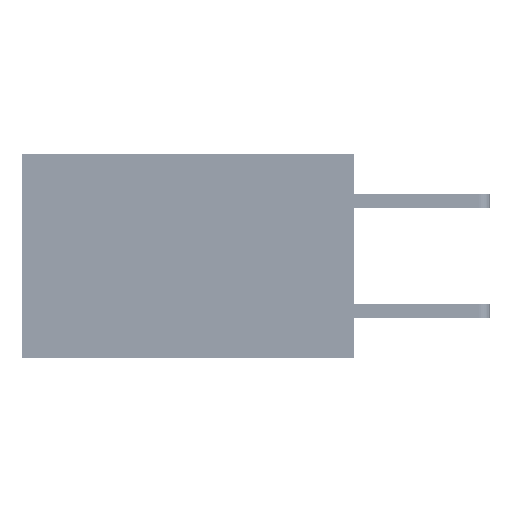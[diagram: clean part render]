
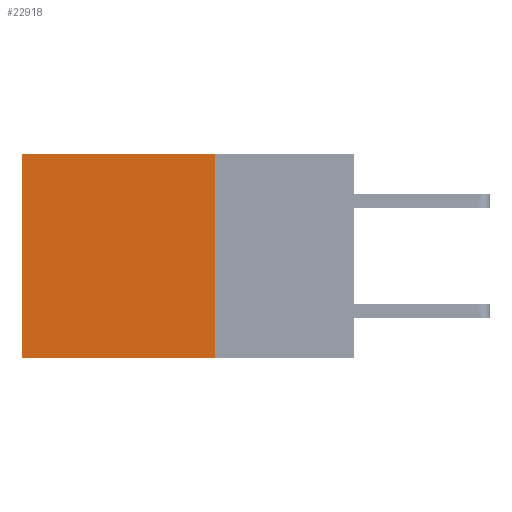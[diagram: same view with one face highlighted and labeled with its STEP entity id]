
A CAD part, left-side view. The second image highlights one B-rep face of the part: STEP entity #22918.
In plain terms, the highlighted planar face has unit normal (-1, 0, 0).
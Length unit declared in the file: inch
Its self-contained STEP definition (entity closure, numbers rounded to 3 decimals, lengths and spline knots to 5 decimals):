
#1767 = VECTOR ( 'NONE', #21073, 39.37008 ) ;
#2287 = VERTEX_POINT ( 'NONE', #46530 ) ;
#2504 = CARTESIAN_POINT ( 'NONE',  ( 0.2875, 0.6, 0. ) ) ;
#5168 = PLANE ( 'NONE',  #28228 ) ;
#5195 = LINE ( 'NONE', #44268, #1767 ) ;
#5915 = DIRECTION ( 'NONE',  ( 1., 0., 0. ) ) ;
#6363 = ORIENTED_EDGE ( 'NONE', *, *, #23171, .T. ) ;
#7543 = ORIENTED_EDGE ( 'NONE', *, *, #28439, .T. ) ;
#7754 = CARTESIAN_POINT ( 'NONE',  ( 0.2875, 0.25, 0. ) ) ;
#10419 = VERTEX_POINT ( 'NONE', #2504 ) ;
#11437 = DIRECTION ( 'NONE',  ( 0., 1., 0. ) ) ;
#13865 = DIRECTION ( 'NONE',  ( 0., 1., 0. ) ) ;
#14761 = VECTOR ( 'NONE', #13865, 39.37008 ) ;
#18818 = CARTESIAN_POINT ( 'NONE',  ( 0.2875, 0.25, 0. ) ) ;
#19521 = CARTESIAN_POINT ( 'NONE',  ( 0.2875, 0.6, -0.37 ) ) ;
#20540 = CARTESIAN_POINT ( 'NONE',  ( 0.2875, 0.25, 0. ) ) ;
#21041 = FACE_OUTER_BOUND ( 'NONE', #22159, .T. ) ;
#21073 = DIRECTION ( 'NONE',  ( 0., 0., -1. ) ) ;
#22159 = EDGE_LOOP ( 'NONE', ( #7543, #45518, #33792, #6363 ) ) ;
#22600 = EDGE_CURVE ( 'NONE', #38400, #2287, #37507, .T. ) ;
#22918 = ADVANCED_FACE ( 'NONE', ( #21041 ), #5168, .F. ) ;
#23171 = EDGE_CURVE ( 'NONE', #38400, #10419, #34877, .T. ) ;
#23288 = CARTESIAN_POINT ( 'NONE',  ( 0.2875, 0.25, 0. ) ) ;
#26338 = EDGE_CURVE ( 'NONE', #2287, #42185, #44632, .T. ) ;
#28228 = AXIS2_PLACEMENT_3D ( 'NONE', #20540, #5915, #28383 ) ;
#28383 = DIRECTION ( 'NONE',  ( 0., 0., -1. ) ) ;
#28439 = EDGE_CURVE ( 'NONE', #10419, #42185, #5195, .T. ) ;
#29773 = CARTESIAN_POINT ( 'NONE',  ( 0.2875, 0.25, -0.37 ) ) ;
#33792 = ORIENTED_EDGE ( 'NONE', *, *, #22600, .F. ) ;
#33903 = VECTOR ( 'NONE', #11437, 39.37008 ) ;
#34198 = DIRECTION ( 'NONE',  ( 0., 0., -1. ) ) ;
#34877 = LINE ( 'NONE', #23288, #33903 ) ;
#37507 = LINE ( 'NONE', #18818, #44336 ) ;
#38400 = VERTEX_POINT ( 'NONE', #7754 ) ;
#42185 = VERTEX_POINT ( 'NONE', #19521 ) ;
#44268 = CARTESIAN_POINT ( 'NONE',  ( 0.2875, 0.6, 0. ) ) ;
#44336 = VECTOR ( 'NONE', #34198, 39.37008 ) ;
#44632 = LINE ( 'NONE', #29773, #14761 ) ;
#45518 = ORIENTED_EDGE ( 'NONE', *, *, #26338, .F. ) ;
#46530 = CARTESIAN_POINT ( 'NONE',  ( 0.2875, 0.25, -0.37 ) ) ;
